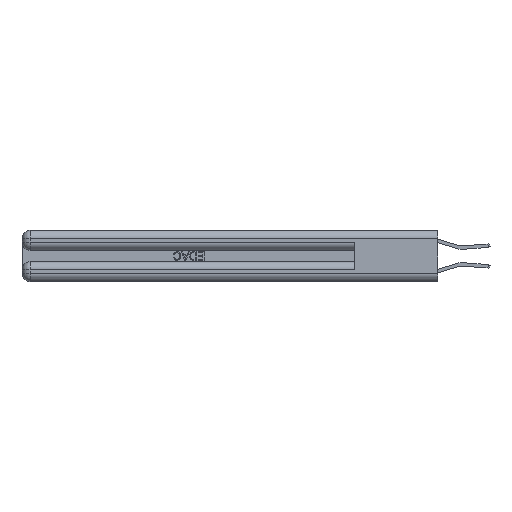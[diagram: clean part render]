
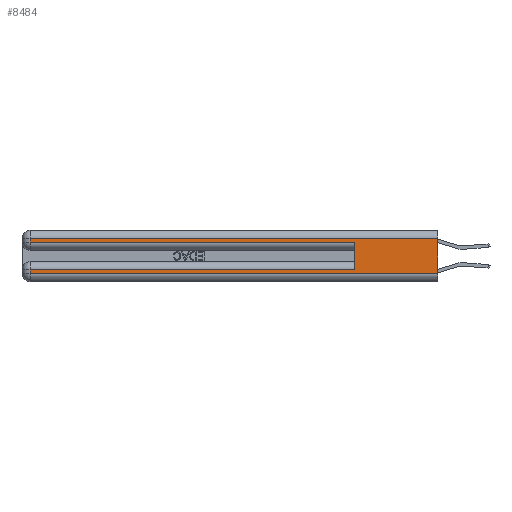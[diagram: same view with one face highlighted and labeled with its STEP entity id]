
A CAD part, left-side view. The second image highlights one B-rep face of the part: STEP entity #8484.
In plain terms, the highlighted planar face has unit normal (-1, 0, 0).
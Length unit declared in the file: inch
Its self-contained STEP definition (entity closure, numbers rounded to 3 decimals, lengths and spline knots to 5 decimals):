
#79 = EDGE_CURVE ( 'NONE', #24341, #26990, #14997, .T. ) ;
#114 = AXIS2_PLACEMENT_3D ( 'NONE', #32703, #21703, #16328 ) ;
#808 = ORIENTED_EDGE ( 'NONE', *, *, #31109, .T. ) ;
#1164 = ORIENTED_EDGE ( 'NONE', *, *, #79, .T. ) ;
#2689 = ORIENTED_EDGE ( 'NONE', *, *, #36746, .T. ) ;
#2783 = CARTESIAN_POINT ( 'NONE',  ( 0., 2.94, 0.085 ) ) ;
#3078 = VERTEX_POINT ( 'NONE', #17054 ) ;
#3747 = VECTOR ( 'NONE', #17094, 39.37008 ) ;
#3970 = CARTESIAN_POINT ( 'NONE',  ( 0., 0.6, 0.085 ) ) ;
#4374 = EDGE_CURVE ( 'NONE', #26990, #33837, #28224, .T. ) ;
#4597 = CARTESIAN_POINT ( 'NONE',  ( 0., 0., 0.06 ) ) ;
#5010 = ORIENTED_EDGE ( 'NONE', *, *, #14998, .T. ) ;
#5147 = DIRECTION ( 'NONE',  ( 0., 0., -1. ) ) ;
#5751 = LINE ( 'NONE', #31805, #35685 ) ;
#6208 = CARTESIAN_POINT ( 'NONE',  ( 0., 0.6, 0.285 ) ) ;
#6868 = ORIENTED_EDGE ( 'NONE', *, *, #31689, .F. ) ;
#7740 = PLANE ( 'NONE',  #114 ) ;
#8304 = DIRECTION ( 'NONE',  ( 0., -1., 0. ) ) ;
#8484 = ADVANCED_FACE ( 'NONE', ( #13161 ), #7740, .F. ) ;
#8523 = CARTESIAN_POINT ( 'NONE',  ( 0., 0., 0.31 ) ) ;
#8527 = EDGE_CURVE ( 'NONE', #3078, #32583, #18745, .T. ) ;
#9017 = CARTESIAN_POINT ( 'NONE',  ( 0., 2.94, 0.285 ) ) ;
#9211 = EDGE_LOOP ( 'NONE', ( #17167, #2689, #1164, #21319, #6868, #5010, #808, #11456 ) ) ;
#9593 = DIRECTION ( 'NONE',  ( 0., 0., -1. ) ) ;
#11456 = ORIENTED_EDGE ( 'NONE', *, *, #8527, .T. ) ;
#11523 = DIRECTION ( 'NONE',  ( 0., 0., 1. ) ) ;
#13161 = FACE_OUTER_BOUND ( 'NONE', #9211, .T. ) ;
#13577 = CARTESIAN_POINT ( 'NONE',  ( 0., 0., 0.085 ) ) ;
#14260 = DIRECTION ( 'NONE',  ( 0., -1., 0. ) ) ;
#14657 = LINE ( 'NONE', #8523, #3747 ) ;
#14997 = LINE ( 'NONE', #35455, #32767 ) ;
#14998 = EDGE_CURVE ( 'NONE', #35341, #18435, #22299, .T. ) ;
#16328 = DIRECTION ( 'NONE',  ( 0., 0., -1. ) ) ;
#16511 = LINE ( 'NONE', #21515, #35064 ) ;
#16785 = VERTEX_POINT ( 'NONE', #20109 ) ;
#17054 = CARTESIAN_POINT ( 'NONE',  ( 0., 2.94, 0.06 ) ) ;
#17094 = DIRECTION ( 'NONE',  ( 0., 1., 0. ) ) ;
#17167 = ORIENTED_EDGE ( 'NONE', *, *, #19892, .F. ) ;
#18435 = VERTEX_POINT ( 'NONE', #2783 ) ;
#18489 = VECTOR ( 'NONE', #8304, 39.37008 ) ;
#18745 = LINE ( 'NONE', #4597, #28644 ) ;
#19157 = DIRECTION ( 'NONE',  ( 0., 1., 0. ) ) ;
#19480 = CARTESIAN_POINT ( 'NONE',  ( 0., 0., 0.285 ) ) ;
#19892 = EDGE_CURVE ( 'NONE', #16785, #32583, #32125, .T. ) ;
#20109 = CARTESIAN_POINT ( 'NONE',  ( 0., 0., 0.31 ) ) ;
#20344 = CARTESIAN_POINT ( 'NONE',  ( 0., 0., 0.06 ) ) ;
#20747 = DIRECTION ( 'NONE',  ( 0., 0., -1. ) ) ;
#21319 = ORIENTED_EDGE ( 'NONE', *, *, #4374, .T. ) ;
#21515 = CARTESIAN_POINT ( 'NONE',  ( 0., 2.94, 0.37 ) ) ;
#21703 = DIRECTION ( 'NONE',  ( 1., 0., 0. ) ) ;
#22299 = LINE ( 'NONE', #13577, #26765 ) ;
#24341 = VERTEX_POINT ( 'NONE', #29061 ) ;
#26765 = VECTOR ( 'NONE', #19157, 39.37008 ) ;
#26990 = VERTEX_POINT ( 'NONE', #9017 ) ;
#28224 = LINE ( 'NONE', #19480, #18489 ) ;
#28644 = VECTOR ( 'NONE', #14260, 39.37008 ) ;
#29061 = CARTESIAN_POINT ( 'NONE',  ( 0., 2.94, 0.31 ) ) ;
#29864 = VECTOR ( 'NONE', #20747, 39.37008 ) ;
#31109 = EDGE_CURVE ( 'NONE', #18435, #3078, #16511, .T. ) ;
#31689 = EDGE_CURVE ( 'NONE', #35341, #33837, #5751, .T. ) ;
#31805 = CARTESIAN_POINT ( 'NONE',  ( 0., 0.6, 0.145 ) ) ;
#32125 = LINE ( 'NONE', #34533, #29864 ) ;
#32583 = VERTEX_POINT ( 'NONE', #20344 ) ;
#32703 = CARTESIAN_POINT ( 'NONE',  ( 0., 0., 0.37 ) ) ;
#32767 = VECTOR ( 'NONE', #9593, 39.37008 ) ;
#33837 = VERTEX_POINT ( 'NONE', #6208 ) ;
#34533 = CARTESIAN_POINT ( 'NONE',  ( 0., 0., 0.37 ) ) ;
#35064 = VECTOR ( 'NONE', #5147, 39.37008 ) ;
#35341 = VERTEX_POINT ( 'NONE', #3970 ) ;
#35455 = CARTESIAN_POINT ( 'NONE',  ( 0., 2.94, 0.37 ) ) ;
#35685 = VECTOR ( 'NONE', #11523, 39.37008 ) ;
#36746 = EDGE_CURVE ( 'NONE', #16785, #24341, #14657, .T. ) ;
